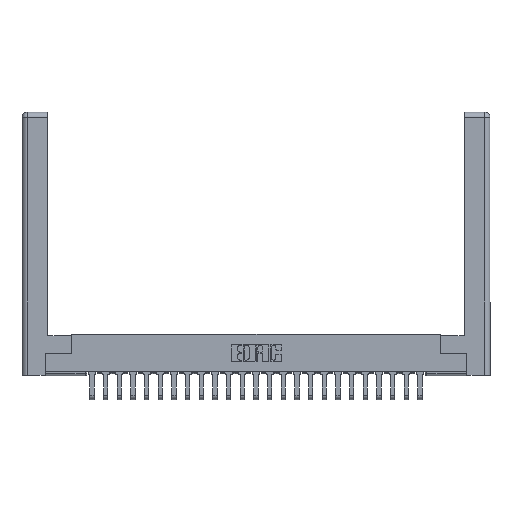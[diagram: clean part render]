
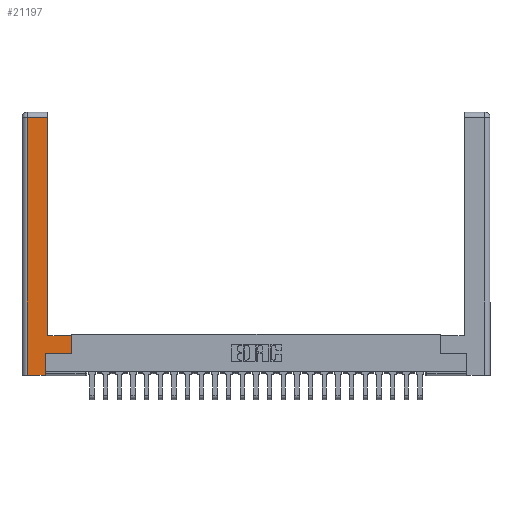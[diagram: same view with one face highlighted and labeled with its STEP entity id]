
A CAD part, top view. The second image highlights one B-rep face of the part: STEP entity #21197.
In plain terms, the highlighted planar face has unit normal (0, 0, 1).
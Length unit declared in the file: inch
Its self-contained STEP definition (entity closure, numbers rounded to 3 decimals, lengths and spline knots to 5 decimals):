
#894 = DIRECTION ( 'NONE',  ( 0., 1., 0. ) ) ;
#946 = LINE ( 'NONE', #14068, #4439 ) ;
#1345 = VECTOR ( 'NONE', #7480, 39.37008 ) ;
#1600 = VERTEX_POINT ( 'NONE', #21922 ) ;
#2081 = DIRECTION ( 'NONE',  ( 0., 1., 0. ) ) ;
#2313 = LINE ( 'NONE', #4891, #7683 ) ;
#2865 = VERTEX_POINT ( 'NONE', #13776 ) ;
#2899 = ORIENTED_EDGE ( 'NONE', *, *, #17194, .T. ) ;
#3292 = CARTESIAN_POINT ( 'NONE',  ( 0.295, 0.45, 0. ) ) ;
#3603 = VERTEX_POINT ( 'NONE', #17001 ) ;
#3927 = EDGE_CURVE ( 'NONE', #2865, #13326, #6724, .T. ) ;
#4242 = CARTESIAN_POINT ( 'NONE',  ( 0.265, 0., 0. ) ) ;
#4399 = LINE ( 'NONE', #16878, #24682 ) ;
#4439 = VECTOR ( 'NONE', #2081, 39.37008 ) ;
#4850 = VECTOR ( 'NONE', #5501, 39.37008 ) ;
#4891 = CARTESIAN_POINT ( 'NONE',  ( 0.0615, 2.94, 0. ) ) ;
#5497 = ORIENTED_EDGE ( 'NONE', *, *, #9874, .T. ) ;
#5501 = DIRECTION ( 'NONE',  ( 1., 0., 0. ) ) ;
#6486 = ORIENTED_EDGE ( 'NONE', *, *, #3927, .T. ) ;
#6588 = VECTOR ( 'NONE', #15782, 39.37008 ) ;
#6601 = CARTESIAN_POINT ( 'NONE',  ( 0.565, 0.245, 0. ) ) ;
#6624 = ORIENTED_EDGE ( 'NONE', *, *, #22157, .T. ) ;
#6724 = LINE ( 'NONE', #11697, #1345 ) ;
#7480 = DIRECTION ( 'NONE',  ( 0., -1., 0. ) ) ;
#7597 = CARTESIAN_POINT ( 'NONE',  ( 0.295, 0.45, 0. ) ) ;
#7683 = VECTOR ( 'NONE', #14656, 39.37008 ) ;
#9213 = CARTESIAN_POINT ( 'NONE',  ( 0., 0., 0. ) ) ;
#9485 = LINE ( 'NONE', #10701, #12699 ) ;
#9874 = EDGE_CURVE ( 'NONE', #23834, #17940, #9485, .T. ) ;
#10448 = DIRECTION ( 'NONE',  ( 0., 1., 0. ) ) ;
#10701 = CARTESIAN_POINT ( 'NONE',  ( 0.265, 0.245, 0. ) ) ;
#11180 = DIRECTION ( 'NONE',  ( 0., 0., -1. ) ) ;
#11416 = EDGE_CURVE ( 'NONE', #1600, #18062, #22491, .T. ) ;
#11697 = CARTESIAN_POINT ( 'NONE',  ( 0.0615, 0., 0. ) ) ;
#12134 = ORIENTED_EDGE ( 'NONE', *, *, #16052, .T. ) ;
#12186 = LINE ( 'NONE', #15365, #4850 ) ;
#12539 = EDGE_CURVE ( 'NONE', #20471, #1600, #4399, .T. ) ;
#12699 = VECTOR ( 'NONE', #10448, 39.37008 ) ;
#12886 = ORIENTED_EDGE ( 'NONE', *, *, #16274, .T. ) ;
#13326 = VERTEX_POINT ( 'NONE', #20558 ) ;
#13776 = CARTESIAN_POINT ( 'NONE',  ( 0.0615, 2.94, 0. ) ) ;
#14068 = CARTESIAN_POINT ( 'NONE',  ( 0.295, 3., 0. ) ) ;
#14656 = DIRECTION ( 'NONE',  ( -1., 0., 0. ) ) ;
#15365 = CARTESIAN_POINT ( 'NONE',  ( 0.565, 0.245, 0. ) ) ;
#15782 = DIRECTION ( 'NONE',  ( -1., 0., 0. ) ) ;
#15917 = LINE ( 'NONE', #4242, #23830 ) ;
#16052 = EDGE_CURVE ( 'NONE', #3603, #2865, #2313, .T. ) ;
#16274 = EDGE_CURVE ( 'NONE', #17940, #20471, #12186, .T. ) ;
#16878 = CARTESIAN_POINT ( 'NONE',  ( 0.565, 0.45, 0. ) ) ;
#17001 = CARTESIAN_POINT ( 'NONE',  ( 0.295, 2.94, 0. ) ) ;
#17119 = PLANE ( 'NONE',  #25289 ) ;
#17194 = EDGE_CURVE ( 'NONE', #13326, #23834, #15917, .T. ) ;
#17940 = VERTEX_POINT ( 'NONE', #23315 ) ;
#18062 = VERTEX_POINT ( 'NONE', #3292 ) ;
#18420 = DIRECTION ( 'NONE',  ( 1., 0., 0. ) ) ;
#20471 = VERTEX_POINT ( 'NONE', #6601 ) ;
#20558 = CARTESIAN_POINT ( 'NONE',  ( 0.0615, 0., 0. ) ) ;
#21197 = ADVANCED_FACE ( 'NONE', ( #21932 ), #17119, .F. ) ;
#21290 = DIRECTION ( 'NONE',  ( -1., 0., 0. ) ) ;
#21879 = ORIENTED_EDGE ( 'NONE', *, *, #11416, .T. ) ;
#21922 = CARTESIAN_POINT ( 'NONE',  ( 0.565, 0.45, 0. ) ) ;
#21932 = FACE_OUTER_BOUND ( 'NONE', #24863, .T. ) ;
#22157 = EDGE_CURVE ( 'NONE', #18062, #3603, #946, .T. ) ;
#22491 = LINE ( 'NONE', #7597, #6588 ) ;
#23315 = CARTESIAN_POINT ( 'NONE',  ( 0.265, 0.245, 0. ) ) ;
#23830 = VECTOR ( 'NONE', #18420, 39.37008 ) ;
#23834 = VERTEX_POINT ( 'NONE', #25756 ) ;
#24131 = ORIENTED_EDGE ( 'NONE', *, *, #12539, .T. ) ;
#24682 = VECTOR ( 'NONE', #894, 39.37008 ) ;
#24863 = EDGE_LOOP ( 'NONE', ( #6624, #12134, #6486, #2899, #5497, #12886, #24131, #21879 ) ) ;
#25289 = AXIS2_PLACEMENT_3D ( 'NONE', #9213, #11180, #21290 ) ;
#25756 = CARTESIAN_POINT ( 'NONE',  ( 0.265, 0., 0. ) ) ;
